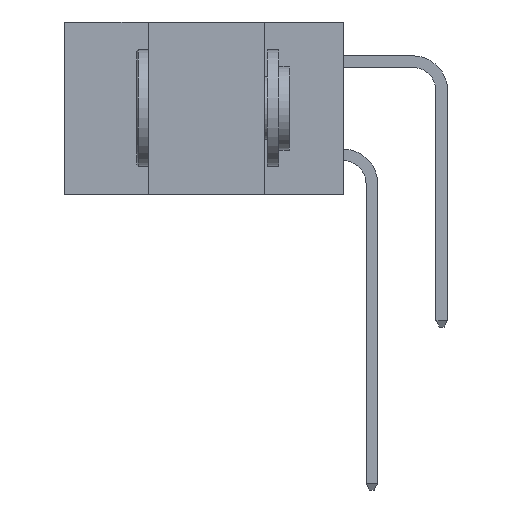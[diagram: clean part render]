
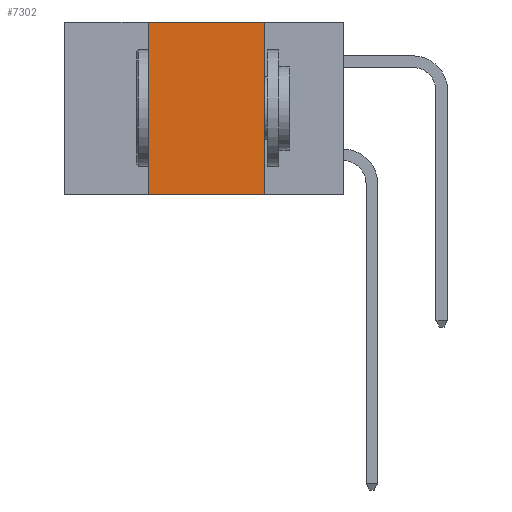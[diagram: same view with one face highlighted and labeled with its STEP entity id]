
A CAD part, left-side view. The second image highlights one B-rep face of the part: STEP entity #7302.
In plain terms, the highlighted planar face has unit normal (-1, 0, 0).
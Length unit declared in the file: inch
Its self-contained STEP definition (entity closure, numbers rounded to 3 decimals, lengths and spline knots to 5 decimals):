
#658 = VECTOR ( 'NONE', #5292, 39.37008 ) ;
#782 = CARTESIAN_POINT ( 'NONE',  ( 0., 0.17, 0. ) ) ;
#2015 = CARTESIAN_POINT ( 'NONE',  ( 0., 0.6, 0. ) ) ;
#2236 = DIRECTION ( 'NONE',  ( 0., 0., 1. ) ) ;
#2474 = CARTESIAN_POINT ( 'NONE',  ( 0., 0.42, -0.37 ) ) ;
#2887 = ORIENTED_EDGE ( 'NONE', *, *, #4358, .F. ) ;
#3081 = EDGE_CURVE ( 'NONE', #12799, #16616, #3675, .T. ) ;
#3528 = DIRECTION ( 'NONE',  ( 0., 0., -1. ) ) ;
#3675 = LINE ( 'NONE', #2474, #7634 ) ;
#3889 = LINE ( 'NONE', #12958, #7389 ) ;
#4358 = EDGE_CURVE ( 'NONE', #16616, #16210, #11992, .T. ) ;
#4571 = CARTESIAN_POINT ( 'NONE',  ( 0., 0.6, -0.37 ) ) ;
#4755 = CARTESIAN_POINT ( 'NONE',  ( 0., 0.42, 0. ) ) ;
#5292 = DIRECTION ( 'NONE',  ( 0., -1., 0. ) ) ;
#5293 = CARTESIAN_POINT ( 'NONE',  ( 0., 0.6, 0. ) ) ;
#5524 = ORIENTED_EDGE ( 'NONE', *, *, #3081, .F. ) ;
#5752 = VECTOR ( 'NONE', #10450, 39.37008 ) ;
#7001 = EDGE_CURVE ( 'NONE', #16210, #11970, #3889, .T. ) ;
#7302 = ADVANCED_FACE ( 'NONE', ( #16768 ), #10844, .F. ) ;
#7328 = ORIENTED_EDGE ( 'NONE', *, *, #7001, .F. ) ;
#7389 = VECTOR ( 'NONE', #17217, 39.37008 ) ;
#7634 = VECTOR ( 'NONE', #2236, 39.37008 ) ;
#8815 = ORIENTED_EDGE ( 'NONE', *, *, #14582, .T. ) ;
#9298 = CARTESIAN_POINT ( 'NONE',  ( 0., 0.42, -0.37 ) ) ;
#10450 = DIRECTION ( 'NONE',  ( 0., -1., 0. ) ) ;
#10844 = PLANE ( 'NONE',  #17899 ) ;
#11970 = VERTEX_POINT ( 'NONE', #18597 ) ;
#11992 = LINE ( 'NONE', #5293, #658 ) ;
#12308 = DIRECTION ( 'NONE',  ( 1., 0., 0. ) ) ;
#12799 = VERTEX_POINT ( 'NONE', #9298 ) ;
#12945 = EDGE_LOOP ( 'NONE', ( #7328, #2887, #5524, #8815 ) ) ;
#12958 = CARTESIAN_POINT ( 'NONE',  ( 0., 0.17, -0.37 ) ) ;
#13880 = LINE ( 'NONE', #4571, #5752 ) ;
#14582 = EDGE_CURVE ( 'NONE', #12799, #11970, #13880, .T. ) ;
#16210 = VERTEX_POINT ( 'NONE', #782 ) ;
#16616 = VERTEX_POINT ( 'NONE', #4755 ) ;
#16768 = FACE_OUTER_BOUND ( 'NONE', #12945, .T. ) ;
#17217 = DIRECTION ( 'NONE',  ( 0., 0., -1. ) ) ;
#17899 = AXIS2_PLACEMENT_3D ( 'NONE', #2015, #12308, #3528 ) ;
#18597 = CARTESIAN_POINT ( 'NONE',  ( 0., 0.17, -0.37 ) ) ;
